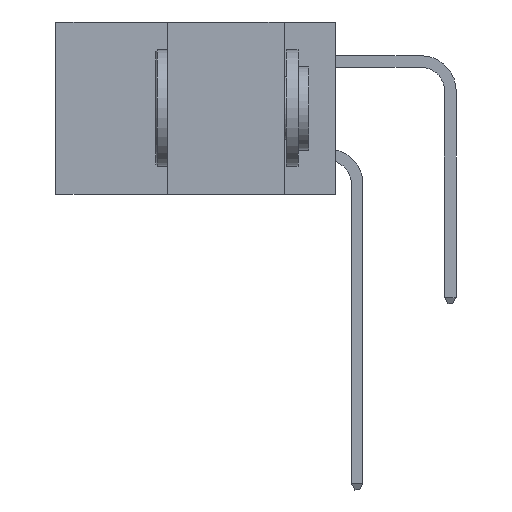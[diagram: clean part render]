
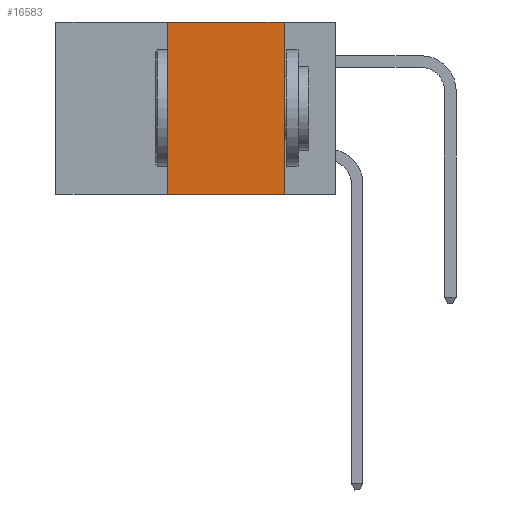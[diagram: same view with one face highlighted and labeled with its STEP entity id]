
A CAD part, left-side view. The second image highlights one B-rep face of the part: STEP entity #16583.
In plain terms, the highlighted planar face has unit normal (-1, 0, 0).
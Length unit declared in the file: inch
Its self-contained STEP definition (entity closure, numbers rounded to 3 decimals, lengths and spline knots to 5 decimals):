
#309 = DIRECTION ( 'NONE',  ( 0., -1., 0. ) ) ;
#330 = CARTESIAN_POINT ( 'NONE',  ( 0., 0.6, 0. ) ) ;
#371 = CARTESIAN_POINT ( 'NONE',  ( 0., 0.36, 0. ) ) ;
#471 = EDGE_CURVE ( 'NONE', #6145, #5057, #5892, .T. ) ;
#1565 = VERTEX_POINT ( 'NONE', #17118 ) ;
#2365 = CARTESIAN_POINT ( 'NONE',  ( 0., 0.36, -0.37 ) ) ;
#2522 = CARTESIAN_POINT ( 'NONE',  ( 0., 0.6, 0. ) ) ;
#2888 = ORIENTED_EDGE ( 'NONE', *, *, #9615, .F. ) ;
#3811 = ORIENTED_EDGE ( 'NONE', *, *, #15112, .F. ) ;
#3940 = DIRECTION ( 'NONE',  ( 0., 0., -1. ) ) ;
#4709 = EDGE_CURVE ( 'NONE', #4716, #1565, #5546, .T. ) ;
#4716 = VERTEX_POINT ( 'NONE', #371 ) ;
#5052 = ORIENTED_EDGE ( 'NONE', *, *, #4709, .F. ) ;
#5057 = VERTEX_POINT ( 'NONE', #5725 ) ;
#5546 = LINE ( 'NONE', #330, #10386 ) ;
#5725 = CARTESIAN_POINT ( 'NONE',  ( 0., 0.11, -0.37 ) ) ;
#5818 = VECTOR ( 'NONE', #13132, 39.37008 ) ;
#5892 = LINE ( 'NONE', #7084, #9478 ) ;
#5972 = ORIENTED_EDGE ( 'NONE', *, *, #471, .T. ) ;
#6145 = VERTEX_POINT ( 'NONE', #2365 ) ;
#6906 = DIRECTION ( 'NONE',  ( 0., 0., 1. ) ) ;
#7070 = DIRECTION ( 'NONE',  ( 0., -1., 0. ) ) ;
#7084 = CARTESIAN_POINT ( 'NONE',  ( 0., 0.6, -0.37 ) ) ;
#9478 = VECTOR ( 'NONE', #7070, 39.37008 ) ;
#9615 = EDGE_CURVE ( 'NONE', #6145, #4716, #10834, .T. ) ;
#10386 = VECTOR ( 'NONE', #309, 39.37008 ) ;
#10653 = PLANE ( 'NONE',  #13186 ) ;
#10834 = LINE ( 'NONE', #16031, #14624 ) ;
#10943 = EDGE_LOOP ( 'NONE', ( #3811, #5052, #2888, #5972 ) ) ;
#11858 = CARTESIAN_POINT ( 'NONE',  ( 0., 0.11, 0. ) ) ;
#11945 = DIRECTION ( 'NONE',  ( 1., 0., 0. ) ) ;
#12445 = LINE ( 'NONE', #11858, #5818 ) ;
#13132 = DIRECTION ( 'NONE',  ( 0., 0., -1. ) ) ;
#13186 = AXIS2_PLACEMENT_3D ( 'NONE', #2522, #11945, #3940 ) ;
#14624 = VECTOR ( 'NONE', #6906, 39.37008 ) ;
#15112 = EDGE_CURVE ( 'NONE', #1565, #5057, #12445, .T. ) ;
#16031 = CARTESIAN_POINT ( 'NONE',  ( 0., 0.36, 0. ) ) ;
#16583 = ADVANCED_FACE ( 'NONE', ( #16784 ), #10653, .F. ) ;
#16784 = FACE_OUTER_BOUND ( 'NONE', #10943, .T. ) ;
#17118 = CARTESIAN_POINT ( 'NONE',  ( 0., 0.11, 0. ) ) ;
